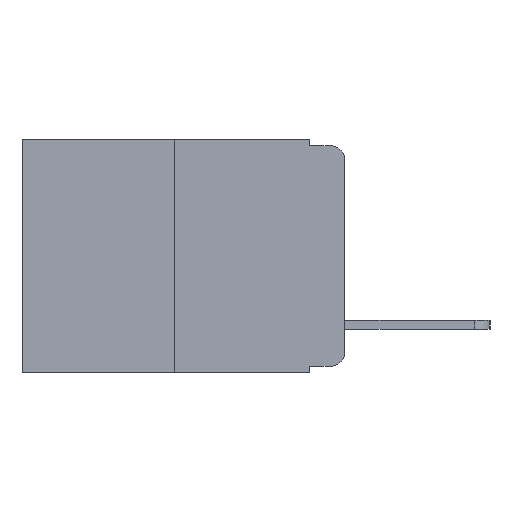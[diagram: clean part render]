
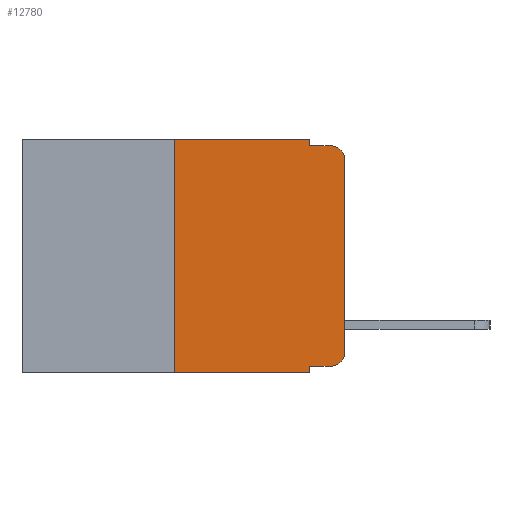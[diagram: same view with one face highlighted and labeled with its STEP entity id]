
A CAD part, left-side view. The second image highlights one B-rep face of the part: STEP entity #12780.
In plain terms, the highlighted planar face has unit normal (-1, 0, 0).
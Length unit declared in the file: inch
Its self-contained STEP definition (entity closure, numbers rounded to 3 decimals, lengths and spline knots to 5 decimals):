
#212 = ORIENTED_EDGE ( 'NONE', *, *, #13218, .F. ) ;
#224 = ORIENTED_EDGE ( 'NONE', *, *, #13232, .T. ) ;
#241 = ORIENTED_EDGE ( 'NONE', *, *, #13216, .F. ) ;
#309 = ORIENTED_EDGE ( 'NONE', *, *, #12739, .T. ) ;
#325 = ORIENTED_EDGE ( 'NONE', *, *, #13192, .F. ) ;
#350 = ORIENTED_EDGE ( 'NONE', *, *, #12298, .F. ) ;
#413 = ORIENTED_EDGE ( 'NONE', *, *, #13169, .T. ) ;
#434 = ORIENTED_EDGE ( 'NONE', *, *, #13190, .F. ) ;
#451 = VERTEX_POINT ( 'NONE', #14231 ) ;
#588 = CIRCLE ( 'NONE', #2996, 0.02 ) ;
#1014 = VECTOR ( 'NONE', #3671, 39.37008 ) ;
#1029 = ORIENTED_EDGE ( 'NONE', *, *, #13234, .T. ) ;
#1190 = CARTESIAN_POINT ( 'NONE',  ( 0., 0., -0.03 ) ) ;
#1468 = LINE ( 'NONE', #12676, #13342 ) ;
#1507 = DIRECTION ( 'NONE',  ( 0., -1., 0. ) ) ;
#2261 = LINE ( 'NONE', #9365, #8331 ) ;
#2335 = CARTESIAN_POINT ( 'NONE',  ( 0., 0.051, 0. ) ) ;
#2396 = CARTESIAN_POINT ( 'NONE',  ( 0., 0.02, -0.01 ) ) ;
#2492 = CARTESIAN_POINT ( 'NONE',  ( 0., 0.25, -0.343 ) ) ;
#2820 = VERTEX_POINT ( 'NONE', #2951 ) ;
#2863 = EDGE_LOOP ( 'NONE', ( #5400, #413, #434, #325, #350, #241, #309, #212, #224, #1029 ) ) ;
#2951 = CARTESIAN_POINT ( 'NONE',  ( 0., 0.051, -0.343 ) ) ;
#2996 = AXIS2_PLACEMENT_3D ( 'NONE', #10685, #3724, #11739 ) ;
#3300 = FACE_OUTER_BOUND ( 'NONE', #2863, .T. ) ;
#3392 = CARTESIAN_POINT ( 'NONE',  ( 0., 0.473, 0. ) ) ;
#3490 = CARTESIAN_POINT ( 'NONE',  ( 0., 0.02, -0.03 ) ) ;
#3671 = DIRECTION ( 'NONE',  ( 0., 0., -1. ) ) ;
#3724 = DIRECTION ( 'NONE',  ( -1., 0., 0. ) ) ;
#4032 = VERTEX_POINT ( 'NONE', #2492 ) ;
#4541 = VERTEX_POINT ( 'NONE', #10370 ) ;
#4623 = DIRECTION ( 'NONE',  ( 0., -1., 0. ) ) ;
#4767 = DIRECTION ( 'NONE',  ( 0., 0., -1. ) ) ;
#4816 = CARTESIAN_POINT ( 'NONE',  ( 0., 0.051, -0.01 ) ) ;
#5283 = CARTESIAN_POINT ( 'NONE',  ( 0., 0.051, -0.333 ) ) ;
#5400 = ORIENTED_EDGE ( 'NONE', *, *, #13168, .T. ) ;
#5614 = LINE ( 'NONE', #4816, #11613 ) ;
#5681 = VERTEX_POINT ( 'NONE', #5283 ) ;
#5854 = DIRECTION ( 'NONE',  ( 0., 0., 1. ) ) ;
#5927 = VERTEX_POINT ( 'NONE', #2396 ) ;
#6048 = CARTESIAN_POINT ( 'NONE',  ( 0., 0.051, -0.333 ) ) ;
#6607 = VERTEX_POINT ( 'NONE', #13910 ) ;
#6936 = CARTESIAN_POINT ( 'NONE',  ( 0., 0.473, -0.343 ) ) ;
#7480 = CARTESIAN_POINT ( 'NONE',  ( 0., 0., -0.313 ) ) ;
#7524 = CARTESIAN_POINT ( 'NONE',  ( 0., 0.051, -0.01 ) ) ;
#7625 = LINE ( 'NONE', #2335, #1014 ) ;
#7845 = LINE ( 'NONE', #12039, #10490 ) ;
#7972 = LINE ( 'NONE', #6048, #10259 ) ;
#8192 = DIRECTION ( 'NONE',  ( 0., 0., -1. ) ) ;
#8331 = VECTOR ( 'NONE', #13623, 39.37008 ) ;
#8368 = DIRECTION ( 'NONE',  ( 0., -1., 0. ) ) ;
#8787 = VERTEX_POINT ( 'NONE', #7524 ) ;
#8984 = CIRCLE ( 'NONE', #11831, 0.02 ) ;
#9191 = VECTOR ( 'NONE', #4623, 39.37008 ) ;
#9341 = VECTOR ( 'NONE', #5854, 39.37008 ) ;
#9365 = CARTESIAN_POINT ( 'NONE',  ( 0., 0.051, 0. ) ) ;
#9467 = DIRECTION ( 'NONE',  ( 0., 0., 1. ) ) ;
#9499 = VERTEX_POINT ( 'NONE', #7480 ) ;
#9674 = VERTEX_POINT ( 'NONE', #1190 ) ;
#9708 = AXIS2_PLACEMENT_3D ( 'NONE', #3392, #14389, #8192 ) ;
#10259 = VECTOR ( 'NONE', #8368, 39.37008 ) ;
#10370 = CARTESIAN_POINT ( 'NONE',  ( 0., 0.02, -0.333 ) ) ;
#10490 = VECTOR ( 'NONE', #1507, 39.37008 ) ;
#10685 = CARTESIAN_POINT ( 'NONE',  ( 0., 0.02, -0.313 ) ) ;
#11564 = DIRECTION ( 'NONE',  ( -1., 0., 0. ) ) ;
#11613 = VECTOR ( 'NONE', #12626, 39.37008 ) ;
#11739 = DIRECTION ( 'NONE',  ( 0., 0., -1. ) ) ;
#11831 = AXIS2_PLACEMENT_3D ( 'NONE', #3490, #11564, #4767 ) ;
#12039 = CARTESIAN_POINT ( 'NONE',  ( 0., 0.473, 0. ) ) ;
#12298 = EDGE_CURVE ( 'NONE', #6607, #451, #7845, .T. ) ;
#12423 = LINE ( 'NONE', #6936, #9191 ) ;
#12626 = DIRECTION ( 'NONE',  ( 0., -1., 0. ) ) ;
#12676 = CARTESIAN_POINT ( 'NONE',  ( 0., 0.25, 0. ) ) ;
#12739 = EDGE_CURVE ( 'NONE', #4032, #2820, #12423, .T. ) ;
#12780 = ADVANCED_FACE ( 'NONE', ( #3300 ), #13508, .F. ) ;
#13168 = EDGE_CURVE ( 'NONE', #9499, #9674, #14442, .T. ) ;
#13169 = EDGE_CURVE ( 'NONE', #9674, #5927, #8984, .T. ) ;
#13190 = EDGE_CURVE ( 'NONE', #8787, #5927, #5614, .T. ) ;
#13192 = EDGE_CURVE ( 'NONE', #451, #8787, #2261, .T. ) ;
#13216 = EDGE_CURVE ( 'NONE', #4032, #6607, #1468, .T. ) ;
#13218 = EDGE_CURVE ( 'NONE', #5681, #2820, #7625, .T. ) ;
#13232 = EDGE_CURVE ( 'NONE', #5681, #4541, #7972, .T. ) ;
#13234 = EDGE_CURVE ( 'NONE', #4541, #9499, #588, .T. ) ;
#13342 = VECTOR ( 'NONE', #9467, 39.37008 ) ;
#13508 = PLANE ( 'NONE',  #9708 ) ;
#13533 = CARTESIAN_POINT ( 'NONE',  ( 0., 0., 0. ) ) ;
#13623 = DIRECTION ( 'NONE',  ( 0., 0., -1. ) ) ;
#13910 = CARTESIAN_POINT ( 'NONE',  ( 0., 0.25, 0. ) ) ;
#14231 = CARTESIAN_POINT ( 'NONE',  ( 0., 0.051, 0. ) ) ;
#14389 = DIRECTION ( 'NONE',  ( 1., 0., 0. ) ) ;
#14442 = LINE ( 'NONE', #13533, #9341 ) ;
